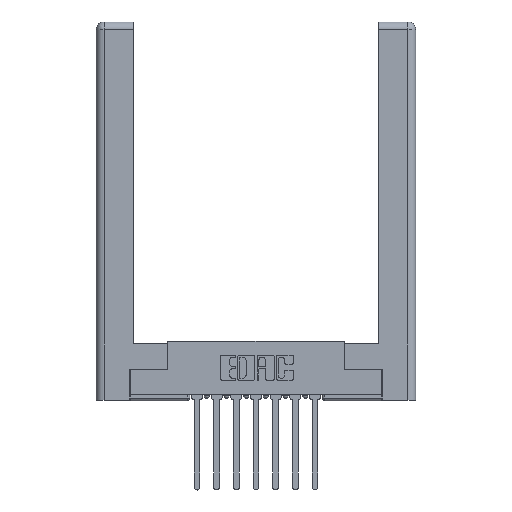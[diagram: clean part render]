
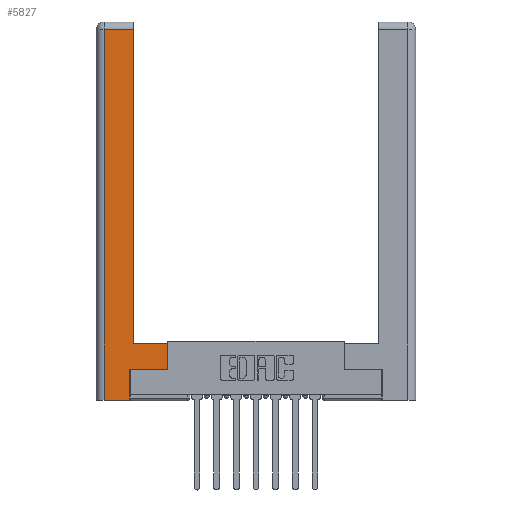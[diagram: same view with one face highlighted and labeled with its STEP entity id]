
A CAD part, top view. The second image highlights one B-rep face of the part: STEP entity #5827.
In plain terms, the highlighted planar face has unit normal (0, 0, 1).
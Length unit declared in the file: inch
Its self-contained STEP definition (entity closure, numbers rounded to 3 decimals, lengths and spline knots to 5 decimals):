
#83 = VERTEX_POINT ( 'NONE', #12518 ) ;
#135 = VECTOR ( 'NONE', #8944, 39.37008 ) ;
#290 = LINE ( 'NONE', #2444, #10604 ) ;
#366 = ORIENTED_EDGE ( 'NONE', *, *, #575, .T. ) ;
#505 = CARTESIAN_POINT ( 'NONE',  ( 0.265, 0.245, 0. ) ) ;
#575 = EDGE_CURVE ( 'NONE', #1770, #4904, #4375, .T. ) ;
#773 = VECTOR ( 'NONE', #2456, 39.37008 ) ;
#812 = VERTEX_POINT ( 'NONE', #2886 ) ;
#894 = EDGE_CURVE ( 'NONE', #5612, #1770, #5296, .T. ) ;
#926 = VECTOR ( 'NONE', #5142, 39.37008 ) ;
#945 = ORIENTED_EDGE ( 'NONE', *, *, #2809, .T. ) ;
#1199 = EDGE_LOOP ( 'NONE', ( #11817, #1269, #945, #11960, #366, #7223, #6401, #12388 ) ) ;
#1207 = LINE ( 'NONE', #6191, #6210 ) ;
#1269 = ORIENTED_EDGE ( 'NONE', *, *, #10176, .T. ) ;
#1632 = CARTESIAN_POINT ( 'NONE',  ( 0.565, 0.245, 0. ) ) ;
#1770 = VERTEX_POINT ( 'NONE', #11630 ) ;
#1934 = FACE_OUTER_BOUND ( 'NONE', #1199, .T. ) ;
#1994 = PLANE ( 'NONE',  #8485 ) ;
#2348 = DIRECTION ( 'NONE',  ( 0., 1., 0. ) ) ;
#2444 = CARTESIAN_POINT ( 'NONE',  ( 0.565, 0.45, 0. ) ) ;
#2456 = DIRECTION ( 'NONE',  ( 0., 1., 0. ) ) ;
#2467 = EDGE_CURVE ( 'NONE', #4904, #7981, #11539, .T. ) ;
#2581 = VECTOR ( 'NONE', #2348, 39.37008 ) ;
#2809 = EDGE_CURVE ( 'NONE', #812, #5612, #1207, .T. ) ;
#2886 = CARTESIAN_POINT ( 'NONE',  ( 0.0615, 2.94, 0. ) ) ;
#3193 = CARTESIAN_POINT ( 'NONE',  ( 0.265, 0., 0. ) ) ;
#4375 = LINE ( 'NONE', #7598, #773 ) ;
#4795 = VECTOR ( 'NONE', #6151, 39.37008 ) ;
#4904 = VERTEX_POINT ( 'NONE', #505 ) ;
#5083 = CARTESIAN_POINT ( 'NONE',  ( 0.565, 0.245, 0. ) ) ;
#5142 = DIRECTION ( 'NONE',  ( 1., 0., 0. ) ) ;
#5296 = LINE ( 'NONE', #3193, #926 ) ;
#5392 = CARTESIAN_POINT ( 'NONE',  ( 0.295, 0.45, 0. ) ) ;
#5612 = VERTEX_POINT ( 'NONE', #9798 ) ;
#5746 = CARTESIAN_POINT ( 'NONE',  ( 0.0615, 2.94, 0. ) ) ;
#5827 = ADVANCED_FACE ( 'NONE', ( #1934 ), #1994, .F. ) ;
#5841 = LINE ( 'NONE', #10196, #2581 ) ;
#6151 = DIRECTION ( 'NONE',  ( -1., 0., 0. ) ) ;
#6183 = DIRECTION ( 'NONE',  ( 0., 1., 0. ) ) ;
#6191 = CARTESIAN_POINT ( 'NONE',  ( 0.0615, 0., 0. ) ) ;
#6210 = VECTOR ( 'NONE', #6314, 39.37008 ) ;
#6314 = DIRECTION ( 'NONE',  ( 0., -1., 0. ) ) ;
#6357 = VECTOR ( 'NONE', #12872, 39.37008 ) ;
#6401 = ORIENTED_EDGE ( 'NONE', *, *, #9357, .T. ) ;
#6573 = VERTEX_POINT ( 'NONE', #5392 ) ;
#6987 = LINE ( 'NONE', #5746, #6357 ) ;
#7223 = ORIENTED_EDGE ( 'NONE', *, *, #2467, .T. ) ;
#7598 = CARTESIAN_POINT ( 'NONE',  ( 0.265, 0.245, 0. ) ) ;
#7981 = VERTEX_POINT ( 'NONE', #5083 ) ;
#8485 = AXIS2_PLACEMENT_3D ( 'NONE', #9460, #12473, #10379 ) ;
#8944 = DIRECTION ( 'NONE',  ( 1., 0., 0. ) ) ;
#9357 = EDGE_CURVE ( 'NONE', #7981, #10260, #290, .T. ) ;
#9460 = CARTESIAN_POINT ( 'NONE',  ( 0., 0., 0. ) ) ;
#9798 = CARTESIAN_POINT ( 'NONE',  ( 0.0615, 0., 0. ) ) ;
#9988 = CARTESIAN_POINT ( 'NONE',  ( 0.565, 0.45, 0. ) ) ;
#10176 = EDGE_CURVE ( 'NONE', #83, #812, #6987, .T. ) ;
#10196 = CARTESIAN_POINT ( 'NONE',  ( 0.295, 3., 0. ) ) ;
#10257 = EDGE_CURVE ( 'NONE', #10260, #6573, #11353, .T. ) ;
#10260 = VERTEX_POINT ( 'NONE', #9988 ) ;
#10379 = DIRECTION ( 'NONE',  ( -1., 0., 0. ) ) ;
#10604 = VECTOR ( 'NONE', #6183, 39.37008 ) ;
#11353 = LINE ( 'NONE', #11995, #4795 ) ;
#11539 = LINE ( 'NONE', #1632, #135 ) ;
#11630 = CARTESIAN_POINT ( 'NONE',  ( 0.265, 0., 0. ) ) ;
#11817 = ORIENTED_EDGE ( 'NONE', *, *, #12244, .T. ) ;
#11960 = ORIENTED_EDGE ( 'NONE', *, *, #894, .T. ) ;
#11995 = CARTESIAN_POINT ( 'NONE',  ( 0.295, 0.45, 0. ) ) ;
#12244 = EDGE_CURVE ( 'NONE', #6573, #83, #5841, .T. ) ;
#12388 = ORIENTED_EDGE ( 'NONE', *, *, #10257, .T. ) ;
#12473 = DIRECTION ( 'NONE',  ( 0., 0., -1. ) ) ;
#12518 = CARTESIAN_POINT ( 'NONE',  ( 0.295, 2.94, 0. ) ) ;
#12872 = DIRECTION ( 'NONE',  ( -1., 0., 0. ) ) ;
